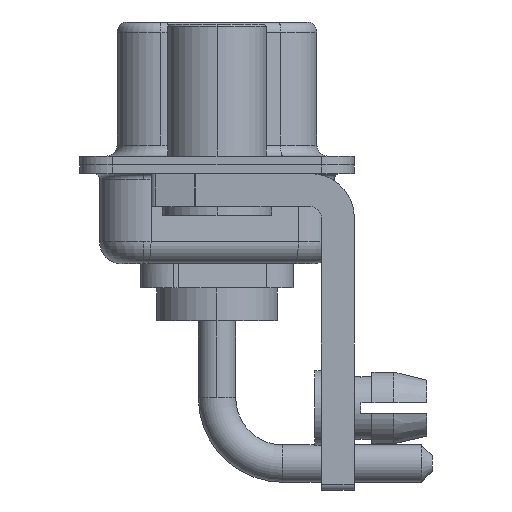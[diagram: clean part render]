
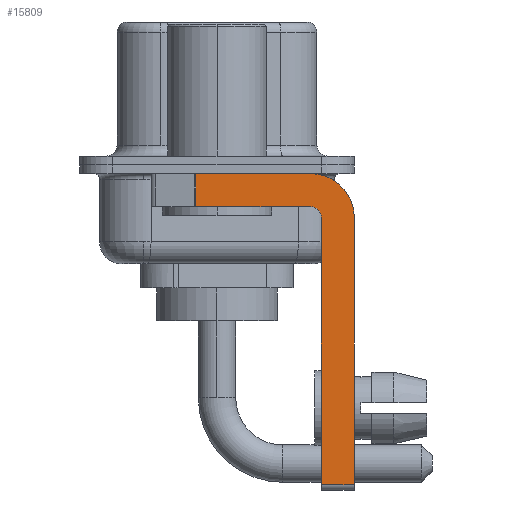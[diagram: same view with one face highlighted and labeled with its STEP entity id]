
A CAD part, left-side view. The second image highlights one B-rep face of the part: STEP entity #15809.
In plain terms, the highlighted planar face has unit normal (-1, 0, 0).
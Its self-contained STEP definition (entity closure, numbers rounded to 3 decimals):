
#66 = ORIENTED_EDGE ( 'NONE', *, *, #9793, .F. ) ;
#72 = VERTEX_POINT ( 'NONE', #18329 ) ;
#252 = EDGE_CURVE ( 'NONE', #7132, #12846, #2351, .T. ) ;
#823 = EDGE_CURVE ( 'NONE', #1281, #1578, #8839, .T. ) ;
#910 = PLANE ( 'NONE',  #16330 ) ;
#1095 = DIRECTION ( 'NONE',  ( 0., -1., 0. ) ) ;
#1281 = VERTEX_POINT ( 'NONE', #18992 ) ;
#1464 = CARTESIAN_POINT ( 'NONE',  ( -2.9, -4.25, -2.4 ) ) ;
#1571 = LINE ( 'NONE', #13648, #3064 ) ;
#1578 = VERTEX_POINT ( 'NONE', #8149 ) ;
#2351 = CIRCLE ( 'NONE', #7413, 0.5 ) ;
#2717 = CARTESIAN_POINT ( 'NONE',  ( -2.9, -4.25, -1.9 ) ) ;
#2807 = VERTEX_POINT ( 'NONE', #18773 ) ;
#3064 = VECTOR ( 'NONE', #18125, 1000. ) ;
#3369 = CIRCLE ( 'NONE', #10641, 2. ) ;
#3454 = CARTESIAN_POINT ( 'NONE',  ( -2.9, -4.25, -2.4 ) ) ;
#3956 = ORIENTED_EDGE ( 'NONE', *, *, #12372, .T. ) ;
#4151 = LINE ( 'NONE', #4247, #5260 ) ;
#4200 = LINE ( 'NONE', #2717, #16954 ) ;
#4247 = CARTESIAN_POINT ( 'NONE',  ( -2.9, -4.75, -14.8 ) ) ;
#4345 = CARTESIAN_POINT ( 'NONE',  ( -2.9, -4.75, -14.55 ) ) ;
#5260 = VECTOR ( 'NONE', #10296, 1000. ) ;
#5458 = ORIENTED_EDGE ( 'NONE', *, *, #823, .F. ) ;
#5602 = DIRECTION ( 'NONE',  ( -1., 0., 0. ) ) ;
#6191 = ORIENTED_EDGE ( 'NONE', *, *, #18911, .F. ) ;
#6545 = CARTESIAN_POINT ( 'NONE',  ( -2.9, -4.75, -2.4 ) ) ;
#6988 = DIRECTION ( 'NONE',  ( 0., 0., 1. ) ) ;
#7132 = VERTEX_POINT ( 'NONE', #6545 ) ;
#7207 = LINE ( 'NONE', #11376, #13460 ) ;
#7413 = AXIS2_PLACEMENT_3D ( 'NONE', #3454, #5602, #6988 ) ;
#8149 = CARTESIAN_POINT ( 'NONE',  ( -2.9, -4.25, -0.4 ) ) ;
#8740 = LINE ( 'NONE', #8837, #17332 ) ;
#8837 = CARTESIAN_POINT ( 'NONE',  ( -2.9, -4.25, -14.55 ) ) ;
#8839 = LINE ( 'NONE', #10422, #14594 ) ;
#9793 = EDGE_CURVE ( 'NONE', #9856, #7132, #4151, .T. ) ;
#9834 = EDGE_CURVE ( 'NONE', #1578, #2807, #3369, .T. ) ;
#9856 = VERTEX_POINT ( 'NONE', #4345 ) ;
#10124 = VERTEX_POINT ( 'NONE', #16008 ) ;
#10142 = FACE_OUTER_BOUND ( 'NONE', #16447, .T. ) ;
#10248 = DIRECTION ( 'NONE',  ( 0., 1., 0. ) ) ;
#10296 = DIRECTION ( 'NONE',  ( 0., 0., 1. ) ) ;
#10422 = CARTESIAN_POINT ( 'NONE',  ( -2.9, 3., -0.4 ) ) ;
#10484 = DIRECTION ( 'NONE',  ( 0., 0., -1. ) ) ;
#10641 = AXIS2_PLACEMENT_3D ( 'NONE', #1464, #16635, #10484 ) ;
#11376 = CARTESIAN_POINT ( 'NONE',  ( -2.9, 0.978, -1.9 ) ) ;
#11631 = DIRECTION ( 'NONE',  ( 1., 0., 0. ) ) ;
#12372 = EDGE_CURVE ( 'NONE', #9856, #72, #8740, .T. ) ;
#12846 = VERTEX_POINT ( 'NONE', #13173 ) ;
#13173 = CARTESIAN_POINT ( 'NONE',  ( -2.9, -4.25, -1.9 ) ) ;
#13244 = DIRECTION ( 'NONE',  ( 0., 0., -1. ) ) ;
#13364 = ORIENTED_EDGE ( 'NONE', *, *, #252, .F. ) ;
#13460 = VECTOR ( 'NONE', #13244, 1000. ) ;
#13648 = CARTESIAN_POINT ( 'NONE',  ( -2.9, -6.25, -2.4 ) ) ;
#14309 = ORIENTED_EDGE ( 'NONE', *, *, #15735, .T. ) ;
#14594 = VECTOR ( 'NONE', #17766, 1000. ) ;
#15299 = ORIENTED_EDGE ( 'NONE', *, *, #9834, .F. ) ;
#15735 = EDGE_CURVE ( 'NONE', #1281, #10124, #7207, .T. ) ;
#15809 = ADVANCED_FACE ( 'NONE', ( #10142 ), #910, .F. ) ;
#16008 = CARTESIAN_POINT ( 'NONE',  ( -2.9, 0.978, -1.9 ) ) ;
#16330 = AXIS2_PLACEMENT_3D ( 'NONE', #19166, #11631, #17471 ) ;
#16447 = EDGE_LOOP ( 'NONE', ( #5458, #14309, #17654, #13364, #66, #3956, #6191, #15299 ) ) ;
#16635 = DIRECTION ( 'NONE',  ( 1., 0., 0. ) ) ;
#16954 = VECTOR ( 'NONE', #10248, 1000. ) ;
#17311 = EDGE_CURVE ( 'NONE', #12846, #10124, #4200, .T. ) ;
#17332 = VECTOR ( 'NONE', #1095, 1000. ) ;
#17471 = DIRECTION ( 'NONE',  ( 0., 0., -1. ) ) ;
#17654 = ORIENTED_EDGE ( 'NONE', *, *, #17311, .F. ) ;
#17766 = DIRECTION ( 'NONE',  ( 0., -1., 0. ) ) ;
#18125 = DIRECTION ( 'NONE',  ( 0., 0., -1. ) ) ;
#18329 = CARTESIAN_POINT ( 'NONE',  ( -2.9, -6.25, -14.55 ) ) ;
#18773 = CARTESIAN_POINT ( 'NONE',  ( -2.9, -6.25, -2.4 ) ) ;
#18911 = EDGE_CURVE ( 'NONE', #2807, #72, #1571, .T. ) ;
#18992 = CARTESIAN_POINT ( 'NONE',  ( -2.9, 0.978, -0.4 ) ) ;
#19166 = CARTESIAN_POINT ( 'NONE',  ( -2.9, -4.25, -2.4 ) ) ;
